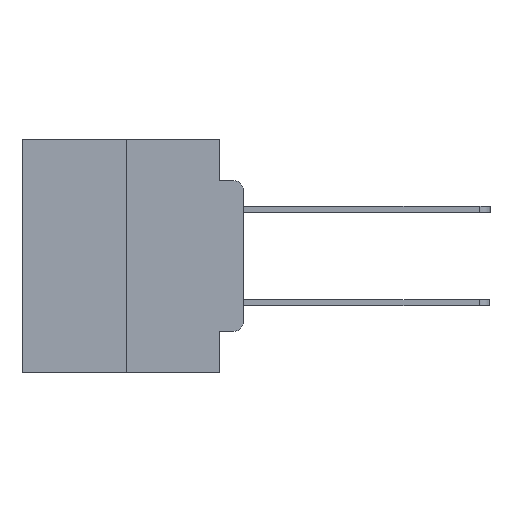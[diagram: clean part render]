
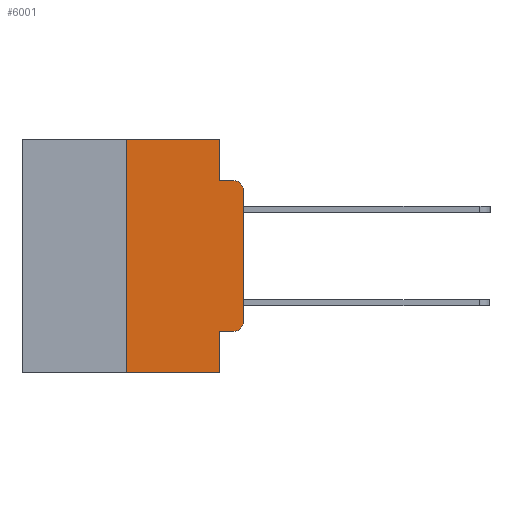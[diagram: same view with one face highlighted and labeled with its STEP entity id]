
A CAD part, left-side view. The second image highlights one B-rep face of the part: STEP entity #6001.
In plain terms, the highlighted planar face has unit normal (-1, 0, 0).
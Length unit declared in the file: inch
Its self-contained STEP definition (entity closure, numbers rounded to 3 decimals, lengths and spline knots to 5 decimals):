
#12 = DIRECTION ( 'NONE',  ( 0., 0., 1. ) ) ;
#74 = CIRCLE ( 'NONE', #22711, 0.02 ) ;
#417 = ORIENTED_EDGE ( 'NONE', *, *, #23414, .F. ) ;
#768 = EDGE_CURVE ( 'NONE', #10493, #5489, #15890, .T. ) ;
#1048 = ORIENTED_EDGE ( 'NONE', *, *, #14103, .F. ) ;
#1628 = VERTEX_POINT ( 'NONE', #12500 ) ;
#1717 = EDGE_CURVE ( 'NONE', #5623, #25630, #20530, .T. ) ;
#2684 = ORIENTED_EDGE ( 'NONE', *, *, #11397, .F. ) ;
#4051 = EDGE_CURVE ( 'NONE', #19347, #1628, #15720, .T. ) ;
#4984 = CARTESIAN_POINT ( 'NONE',  ( 0., 0.051, -0.4115 ) ) ;
#5242 = CARTESIAN_POINT ( 'NONE',  ( 0., 0.051, -0.5 ) ) ;
#5489 = VERTEX_POINT ( 'NONE', #23911 ) ;
#5623 = VERTEX_POINT ( 'NONE', #4984 ) ;
#5660 = CARTESIAN_POINT ( 'NONE',  ( 0., 0.02, -0.3915 ) ) ;
#6001 = ADVANCED_FACE ( 'NONE', ( #10514 ), #13638, .F. ) ;
#6051 = DIRECTION ( 'NONE',  ( 0., -1., 0. ) ) ;
#6312 = CARTESIAN_POINT ( 'NONE',  ( 0., 0.051, -0.4115 ) ) ;
#6336 = VERTEX_POINT ( 'NONE', #20759 ) ;
#6674 = CARTESIAN_POINT ( 'NONE',  ( 0., 0.051, -0.0885 ) ) ;
#6742 = LINE ( 'NONE', #20964, #17470 ) ;
#6765 = CARTESIAN_POINT ( 'NONE',  ( 0., 0.25, 0. ) ) ;
#7205 = AXIS2_PLACEMENT_3D ( 'NONE', #9301, #23260, #11332 ) ;
#7325 = EDGE_CURVE ( 'NONE', #25630, #6336, #74, .T. ) ;
#7331 = ORIENTED_EDGE ( 'NONE', *, *, #8190, .T. ) ;
#7608 = CARTESIAN_POINT ( 'NONE',  ( 0., 0.473, 0. ) ) ;
#7727 = DIRECTION ( 'NONE',  ( 0., 0., -1. ) ) ;
#7923 = ORIENTED_EDGE ( 'NONE', *, *, #18141, .F. ) ;
#7992 = LINE ( 'NONE', #24199, #24548 ) ;
#8190 = EDGE_CURVE ( 'NONE', #6336, #19347, #17617, .T. ) ;
#8583 = CARTESIAN_POINT ( 'NONE',  ( 0., 0., -0.1085 ) ) ;
#9194 = VECTOR ( 'NONE', #18752, 39.37008 ) ;
#9301 = CARTESIAN_POINT ( 'NONE',  ( 0., 0.02, -0.1085 ) ) ;
#9646 = DIRECTION ( 'NONE',  ( 1., 0., 0. ) ) ;
#9830 = LINE ( 'NONE', #6674, #9194 ) ;
#9941 = VECTOR ( 'NONE', #20825, 39.37008 ) ;
#10493 = VERTEX_POINT ( 'NONE', #21981 ) ;
#10498 = VECTOR ( 'NONE', #6051, 39.37008 ) ;
#10514 = FACE_OUTER_BOUND ( 'NONE', #19551, .T. ) ;
#10553 = VECTOR ( 'NONE', #18480, 39.37008 ) ;
#10839 = VERTEX_POINT ( 'NONE', #23068 ) ;
#11332 = DIRECTION ( 'NONE',  ( 0., 0., -1. ) ) ;
#11397 = EDGE_CURVE ( 'NONE', #10839, #10493, #15280, .T. ) ;
#12277 = CARTESIAN_POINT ( 'NONE',  ( 0., 0., 0. ) ) ;
#12278 = DIRECTION ( 'NONE',  ( 0., 0., -1. ) ) ;
#12322 = LINE ( 'NONE', #17482, #22308 ) ;
#12500 = CARTESIAN_POINT ( 'NONE',  ( 0., 0.02, -0.0885 ) ) ;
#13038 = DIRECTION ( 'NONE',  ( 0., -1., 0. ) ) ;
#13101 = ORIENTED_EDGE ( 'NONE', *, *, #7325, .T. ) ;
#13477 = DIRECTION ( 'NONE',  ( 0., 0., -1. ) ) ;
#13638 = PLANE ( 'NONE',  #20376 ) ;
#13976 = CARTESIAN_POINT ( 'NONE',  ( 0., 0.051, -0.0885 ) ) ;
#14103 = EDGE_CURVE ( 'NONE', #5623, #25520, #12322, .T. ) ;
#15169 = ORIENTED_EDGE ( 'NONE', *, *, #4051, .T. ) ;
#15280 = LINE ( 'NONE', #6765, #9941 ) ;
#15720 = CIRCLE ( 'NONE', #7205, 0.02 ) ;
#15890 = LINE ( 'NONE', #16186, #10553 ) ;
#16186 = CARTESIAN_POINT ( 'NONE',  ( 0., 0.473, 0. ) ) ;
#16352 = VECTOR ( 'NONE', #12, 39.37008 ) ;
#17470 = VECTOR ( 'NONE', #13038, 39.37008 ) ;
#17482 = CARTESIAN_POINT ( 'NONE',  ( 0., 0.051, 0. ) ) ;
#17617 = LINE ( 'NONE', #12277, #16352 ) ;
#18141 = EDGE_CURVE ( 'NONE', #23330, #1628, #9830, .T. ) ;
#18480 = DIRECTION ( 'NONE',  ( 0., -1., 0. ) ) ;
#18752 = DIRECTION ( 'NONE',  ( 0., -1., 0. ) ) ;
#19347 = VERTEX_POINT ( 'NONE', #8583 ) ;
#19551 = EDGE_LOOP ( 'NONE', ( #7331, #15169, #7923, #417, #19553, #2684, #23539, #1048, #19679, #13101 ) ) ;
#19553 = ORIENTED_EDGE ( 'NONE', *, *, #768, .F. ) ;
#19634 = CARTESIAN_POINT ( 'NONE',  ( 0., 0.02, -0.4115 ) ) ;
#19679 = ORIENTED_EDGE ( 'NONE', *, *, #1717, .T. ) ;
#19770 = DIRECTION ( 'NONE',  ( -1., 0., 0. ) ) ;
#20376 = AXIS2_PLACEMENT_3D ( 'NONE', #7608, #9646, #23597 ) ;
#20530 = LINE ( 'NONE', #6312, #10498 ) ;
#20759 = CARTESIAN_POINT ( 'NONE',  ( 0., 0., -0.3915 ) ) ;
#20825 = DIRECTION ( 'NONE',  ( 0., 0., 1. ) ) ;
#20964 = CARTESIAN_POINT ( 'NONE',  ( 0., 0.473, -0.5 ) ) ;
#21981 = CARTESIAN_POINT ( 'NONE',  ( 0., 0.25, 0. ) ) ;
#22308 = VECTOR ( 'NONE', #13477, 39.37008 ) ;
#22632 = EDGE_CURVE ( 'NONE', #10839, #25520, #6742, .T. ) ;
#22711 = AXIS2_PLACEMENT_3D ( 'NONE', #5660, #19770, #7727 ) ;
#23068 = CARTESIAN_POINT ( 'NONE',  ( 0., 0.25, -0.5 ) ) ;
#23260 = DIRECTION ( 'NONE',  ( -1., 0., 0. ) ) ;
#23330 = VERTEX_POINT ( 'NONE', #13976 ) ;
#23414 = EDGE_CURVE ( 'NONE', #5489, #23330, #7992, .T. ) ;
#23539 = ORIENTED_EDGE ( 'NONE', *, *, #22632, .T. ) ;
#23597 = DIRECTION ( 'NONE',  ( 0., 0., -1. ) ) ;
#23911 = CARTESIAN_POINT ( 'NONE',  ( 0., 0.051, 0. ) ) ;
#24199 = CARTESIAN_POINT ( 'NONE',  ( 0., 0.051, 0. ) ) ;
#24548 = VECTOR ( 'NONE', #12278, 39.37008 ) ;
#25520 = VERTEX_POINT ( 'NONE', #5242 ) ;
#25630 = VERTEX_POINT ( 'NONE', #19634 ) ;
